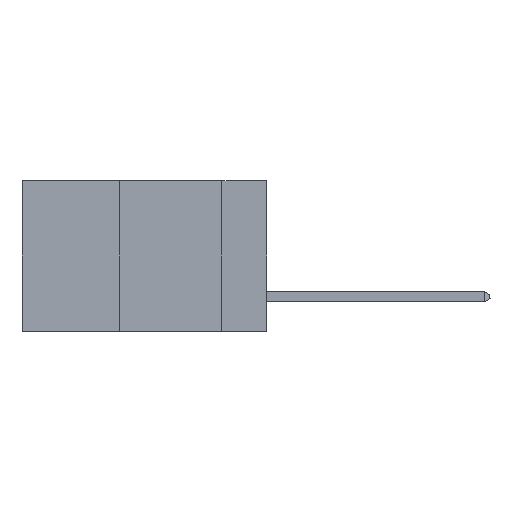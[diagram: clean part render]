
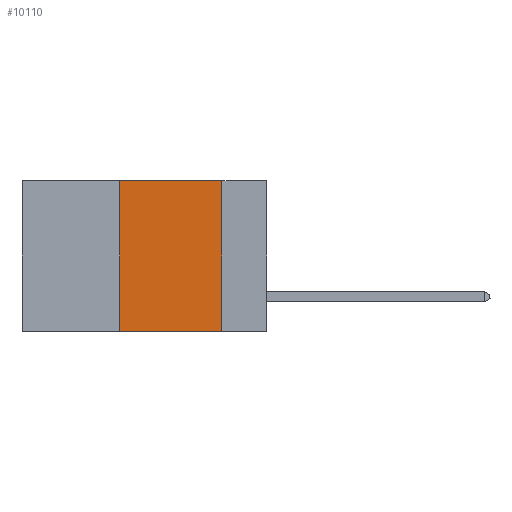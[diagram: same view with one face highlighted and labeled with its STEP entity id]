
A CAD part, left-side view. The second image highlights one B-rep face of the part: STEP entity #10110.
In plain terms, the highlighted planar face has unit normal (-1, 0, 0).
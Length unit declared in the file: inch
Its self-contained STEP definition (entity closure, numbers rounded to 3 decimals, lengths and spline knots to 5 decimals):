
#468 = DIRECTION ( 'NONE',  ( 0., -1., 0. ) ) ;
#566 = CARTESIAN_POINT ( 'NONE',  ( 0., 0.6, 0. ) ) ;
#1005 = LINE ( 'NONE', #12859, #15082 ) ;
#1180 = ORIENTED_EDGE ( 'NONE', *, *, #1223, .F. ) ;
#1223 = EDGE_CURVE ( 'NONE', #11331, #16946, #18995, .T. ) ;
#1398 = CARTESIAN_POINT ( 'NONE',  ( 0., 0.11, 0. ) ) ;
#1761 = VECTOR ( 'NONE', #7589, 39.37008 ) ;
#1926 = FACE_OUTER_BOUND ( 'NONE', #3455, .T. ) ;
#2134 = DIRECTION ( 'NONE',  ( 0., 0., -1. ) ) ;
#2175 = AXIS2_PLACEMENT_3D ( 'NONE', #566, #13614, #2134 ) ;
#2919 = CARTESIAN_POINT ( 'NONE',  ( 0., 0.11, -0.37 ) ) ;
#3366 = VERTEX_POINT ( 'NONE', #1398 ) ;
#3455 = EDGE_LOOP ( 'NONE', ( #4040, #17287, #1180, #18523 ) ) ;
#4040 = ORIENTED_EDGE ( 'NONE', *, *, #18072, .F. ) ;
#4325 = VECTOR ( 'NONE', #11560, 39.37008 ) ;
#6215 = CARTESIAN_POINT ( 'NONE',  ( 0., 0.36, -0.37 ) ) ;
#7589 = DIRECTION ( 'NONE',  ( 0., 0., -1. ) ) ;
#8059 = CARTESIAN_POINT ( 'NONE',  ( 0., 0.36, 0. ) ) ;
#8081 = DIRECTION ( 'NONE',  ( 0., -1., 0. ) ) ;
#9444 = CARTESIAN_POINT ( 'NONE',  ( 0., 0.11, 0. ) ) ;
#10110 = ADVANCED_FACE ( 'NONE', ( #1926 ), #20138, .F. ) ;
#11331 = VERTEX_POINT ( 'NONE', #6215 ) ;
#11560 = DIRECTION ( 'NONE',  ( 0., 0., 1. ) ) ;
#12749 = VERTEX_POINT ( 'NONE', #2919 ) ;
#12859 = CARTESIAN_POINT ( 'NONE',  ( 0., 0.6, 0. ) ) ;
#13614 = DIRECTION ( 'NONE',  ( 1., 0., 0. ) ) ;
#14326 = LINE ( 'NONE', #9444, #1761 ) ;
#15082 = VECTOR ( 'NONE', #8081, 39.37008 ) ;
#15958 = EDGE_CURVE ( 'NONE', #11331, #12749, #19023, .T. ) ;
#16197 = VECTOR ( 'NONE', #468, 39.37008 ) ;
#16343 = EDGE_CURVE ( 'NONE', #16946, #3366, #1005, .T. ) ;
#16858 = CARTESIAN_POINT ( 'NONE',  ( 0., 0.36, 0. ) ) ;
#16946 = VERTEX_POINT ( 'NONE', #8059 ) ;
#17287 = ORIENTED_EDGE ( 'NONE', *, *, #16343, .F. ) ;
#18072 = EDGE_CURVE ( 'NONE', #3366, #12749, #14326, .T. ) ;
#18523 = ORIENTED_EDGE ( 'NONE', *, *, #15958, .T. ) ;
#18714 = CARTESIAN_POINT ( 'NONE',  ( 0., 0.6, -0.37 ) ) ;
#18995 = LINE ( 'NONE', #16858, #4325 ) ;
#19023 = LINE ( 'NONE', #18714, #16197 ) ;
#20138 = PLANE ( 'NONE',  #2175 ) ;
